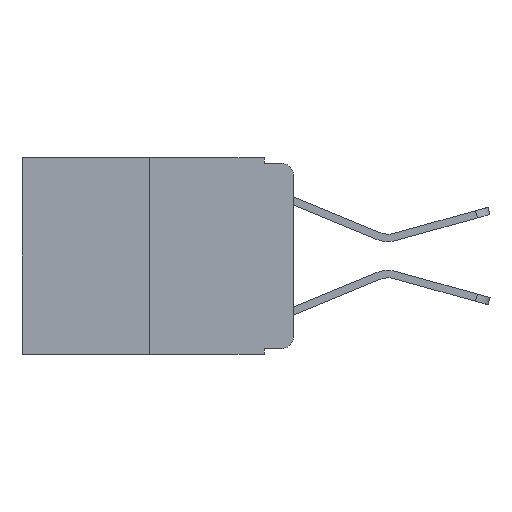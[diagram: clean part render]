
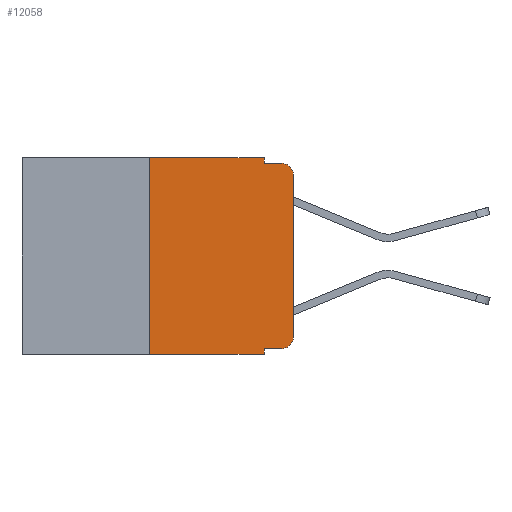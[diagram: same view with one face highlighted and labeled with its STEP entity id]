
A CAD part, left-side view. The second image highlights one B-rep face of the part: STEP entity #12058.
In plain terms, the highlighted planar face has unit normal (-1, 0, 0).
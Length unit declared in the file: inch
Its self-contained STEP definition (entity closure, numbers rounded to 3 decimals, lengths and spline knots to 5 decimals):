
#127 = VERTEX_POINT ( 'NONE', #2356 ) ;
#302 = DIRECTION ( 'NONE',  ( 0., -1., 0. ) ) ;
#652 = LINE ( 'NONE', #3474, #11663 ) ;
#1274 = VECTOR ( 'NONE', #2404, 39.37008 ) ;
#1278 = DIRECTION ( 'NONE',  ( 0., 0., -1. ) ) ;
#1802 = FACE_OUTER_BOUND ( 'NONE', #6294, .T. ) ;
#2037 = CARTESIAN_POINT ( 'NONE',  ( 0., 0.25, -0.343 ) ) ;
#2173 = EDGE_CURVE ( 'NONE', #127, #2662, #9463, .T. ) ;
#2356 = CARTESIAN_POINT ( 'NONE',  ( 0., 0.02, -0.333 ) ) ;
#2362 = DIRECTION ( 'NONE',  ( 0., -1., 0. ) ) ;
#2404 = DIRECTION ( 'NONE',  ( 0., 0., 1. ) ) ;
#2442 = EDGE_CURVE ( 'NONE', #7230, #13790, #4058, .T. ) ;
#2480 = ORIENTED_EDGE ( 'NONE', *, *, #5068, .T. ) ;
#2662 = VERTEX_POINT ( 'NONE', #9299 ) ;
#2986 = CARTESIAN_POINT ( 'NONE',  ( 0., 0.473, 0. ) ) ;
#3252 = DIRECTION ( 'NONE',  ( 0., 0., -1. ) ) ;
#3474 = CARTESIAN_POINT ( 'NONE',  ( 0., 0.051, -0.333 ) ) ;
#4003 = VERTEX_POINT ( 'NONE', #5267 ) ;
#4058 = LINE ( 'NONE', #9013, #10057 ) ;
#4385 = CARTESIAN_POINT ( 'NONE',  ( 0., 0.051, 0. ) ) ;
#4387 = PLANE ( 'NONE',  #16564 ) ;
#4741 = DIRECTION ( 'NONE',  ( 0., 0., -1. ) ) ;
#5068 = EDGE_CURVE ( 'NONE', #2662, #4003, #9356, .T. ) ;
#5267 = CARTESIAN_POINT ( 'NONE',  ( 0., 0., -0.03 ) ) ;
#5343 = CARTESIAN_POINT ( 'NONE',  ( 0., 0.02, -0.01 ) ) ;
#5614 = LINE ( 'NONE', #4385, #10772 ) ;
#5663 = DIRECTION ( 'NONE',  ( 0., 0., -1. ) ) ;
#5719 = DIRECTION ( 'NONE',  ( 0., 0., -1. ) ) ;
#5801 = CARTESIAN_POINT ( 'NONE',  ( 0., 0.051, -0.01 ) ) ;
#6213 = DIRECTION ( 'NONE',  ( 0., 0., 1. ) ) ;
#6294 = EDGE_LOOP ( 'NONE', ( #2480, #6887, #15565, #10294, #8930, #8296, #15323, #6440, #7153, #8752 ) ) ;
#6440 = ORIENTED_EDGE ( 'NONE', *, *, #2442, .F. ) ;
#6701 = VERTEX_POINT ( 'NONE', #12048 ) ;
#6757 = VECTOR ( 'NONE', #12032, 39.37008 ) ;
#6885 = LINE ( 'NONE', #7314, #12873 ) ;
#6887 = ORIENTED_EDGE ( 'NONE', *, *, #15731, .T. ) ;
#6906 = LINE ( 'NONE', #5801, #9182 ) ;
#7112 = CARTESIAN_POINT ( 'NONE',  ( 0., 0.02, -0.313 ) ) ;
#7153 = ORIENTED_EDGE ( 'NONE', *, *, #14291, .T. ) ;
#7193 = VERTEX_POINT ( 'NONE', #14455 ) ;
#7230 = VERTEX_POINT ( 'NONE', #14573 ) ;
#7314 = CARTESIAN_POINT ( 'NONE',  ( 0., 0.25, 0. ) ) ;
#7512 = CIRCLE ( 'NONE', #14614, 0.02 ) ;
#7966 = AXIS2_PLACEMENT_3D ( 'NONE', #7112, #13785, #3252 ) ;
#8296 = ORIENTED_EDGE ( 'NONE', *, *, #10170, .F. ) ;
#8452 = EDGE_CURVE ( 'NONE', #16893, #6701, #9025, .T. ) ;
#8752 = ORIENTED_EDGE ( 'NONE', *, *, #2173, .T. ) ;
#8827 = VERTEX_POINT ( 'NONE', #5343 ) ;
#8930 = ORIENTED_EDGE ( 'NONE', *, *, #8452, .F. ) ;
#8988 = CARTESIAN_POINT ( 'NONE',  ( 0., 0.473, -0.343 ) ) ;
#9013 = CARTESIAN_POINT ( 'NONE',  ( 0., 0.051, 0. ) ) ;
#9025 = LINE ( 'NONE', #10812, #6757 ) ;
#9182 = VECTOR ( 'NONE', #302, 39.37008 ) ;
#9299 = CARTESIAN_POINT ( 'NONE',  ( 0., 0., -0.313 ) ) ;
#9356 = LINE ( 'NONE', #16719, #1274 ) ;
#9359 = VECTOR ( 'NONE', #2362, 39.37008 ) ;
#9463 = CIRCLE ( 'NONE', #7966, 0.02 ) ;
#10057 = VECTOR ( 'NONE', #1278, 39.37008 ) ;
#10170 = EDGE_CURVE ( 'NONE', #16606, #16893, #6885, .T. ) ;
#10294 = ORIENTED_EDGE ( 'NONE', *, *, #15959, .F. ) ;
#10356 = EDGE_CURVE ( 'NONE', #16606, #13790, #15981, .T. ) ;
#10772 = VECTOR ( 'NONE', #5719, 39.37008 ) ;
#10812 = CARTESIAN_POINT ( 'NONE',  ( 0., 0.473, 0. ) ) ;
#11663 = VECTOR ( 'NONE', #16976, 39.37008 ) ;
#12032 = DIRECTION ( 'NONE',  ( 0., -1., 0. ) ) ;
#12048 = CARTESIAN_POINT ( 'NONE',  ( 0., 0.051, 0. ) ) ;
#12058 = ADVANCED_FACE ( 'NONE', ( #1802 ), #4387, .F. ) ;
#12192 = CARTESIAN_POINT ( 'NONE',  ( 0., 0.02, -0.03 ) ) ;
#12250 = DIRECTION ( 'NONE',  ( -1., 0., 0. ) ) ;
#12873 = VECTOR ( 'NONE', #6213, 39.37008 ) ;
#13785 = DIRECTION ( 'NONE',  ( -1., 0., 0. ) ) ;
#13790 = VERTEX_POINT ( 'NONE', #16858 ) ;
#14291 = EDGE_CURVE ( 'NONE', #7230, #127, #652, .T. ) ;
#14455 = CARTESIAN_POINT ( 'NONE',  ( 0., 0.051, -0.01 ) ) ;
#14573 = CARTESIAN_POINT ( 'NONE',  ( 0., 0.051, -0.333 ) ) ;
#14614 = AXIS2_PLACEMENT_3D ( 'NONE', #12192, #12250, #5663 ) ;
#14650 = CARTESIAN_POINT ( 'NONE',  ( 0., 0.25, 0. ) ) ;
#14971 = DIRECTION ( 'NONE',  ( 1., 0., 0. ) ) ;
#15190 = EDGE_CURVE ( 'NONE', #7193, #8827, #6906, .T. ) ;
#15323 = ORIENTED_EDGE ( 'NONE', *, *, #10356, .T. ) ;
#15565 = ORIENTED_EDGE ( 'NONE', *, *, #15190, .F. ) ;
#15731 = EDGE_CURVE ( 'NONE', #4003, #8827, #7512, .T. ) ;
#15959 = EDGE_CURVE ( 'NONE', #6701, #7193, #5614, .T. ) ;
#15981 = LINE ( 'NONE', #8988, #9359 ) ;
#16564 = AXIS2_PLACEMENT_3D ( 'NONE', #2986, #14971, #4741 ) ;
#16606 = VERTEX_POINT ( 'NONE', #2037 ) ;
#16719 = CARTESIAN_POINT ( 'NONE',  ( 0., 0., 0. ) ) ;
#16858 = CARTESIAN_POINT ( 'NONE',  ( 0., 0.051, -0.343 ) ) ;
#16893 = VERTEX_POINT ( 'NONE', #14650 ) ;
#16976 = DIRECTION ( 'NONE',  ( 0., -1., 0. ) ) ;
